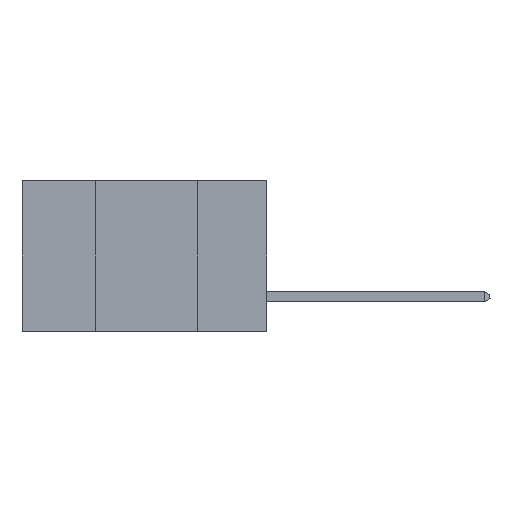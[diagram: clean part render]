
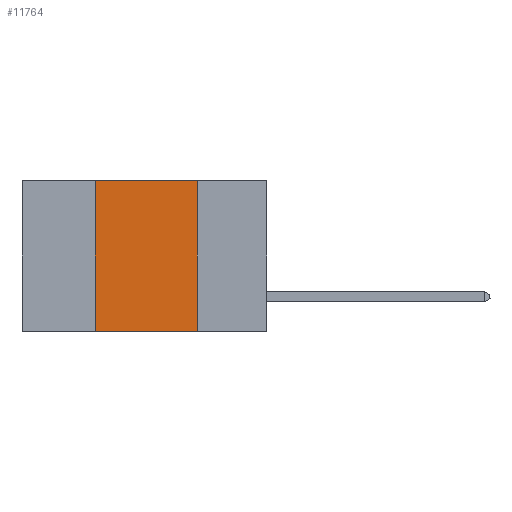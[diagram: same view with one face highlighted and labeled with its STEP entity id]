
A CAD part, left-side view. The second image highlights one B-rep face of the part: STEP entity #11764.
In plain terms, the highlighted planar face has unit normal (-1, 0, 0).
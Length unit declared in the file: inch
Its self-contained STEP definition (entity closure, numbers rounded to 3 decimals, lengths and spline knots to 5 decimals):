
#420 = PLANE ( 'NONE',  #907 ) ;
#666 = VECTOR ( 'NONE', #4192, 39.37008 ) ;
#707 = EDGE_CURVE ( 'NONE', #9899, #2850, #5835, .T. ) ;
#907 = AXIS2_PLACEMENT_3D ( 'NONE', #1849, #9413, #3931 ) ;
#1086 = ORIENTED_EDGE ( 'NONE', *, *, #3084, .F. ) ;
#1494 = EDGE_CURVE ( 'NONE', #9899, #6217, #3956, .T. ) ;
#1543 = EDGE_CURVE ( 'NONE', #2850, #6375, #12144, .T. ) ;
#1849 = CARTESIAN_POINT ( 'NONE',  ( 0., 0.6, 0. ) ) ;
#1938 = VECTOR ( 'NONE', #7849, 39.37008 ) ;
#2269 = CARTESIAN_POINT ( 'NONE',  ( 0., 0.6, -0.37 ) ) ;
#2850 = VERTEX_POINT ( 'NONE', #7704 ) ;
#2855 = CARTESIAN_POINT ( 'NONE',  ( 0., 0.17, 0. ) ) ;
#3084 = EDGE_CURVE ( 'NONE', #6375, #6217, #12260, .T. ) ;
#3342 = ORIENTED_EDGE ( 'NONE', *, *, #1494, .T. ) ;
#3931 = DIRECTION ( 'NONE',  ( 0., 0., -1. ) ) ;
#3956 = LINE ( 'NONE', #2269, #666 ) ;
#4192 = DIRECTION ( 'NONE',  ( 0., -1., 0. ) ) ;
#5398 = ORIENTED_EDGE ( 'NONE', *, *, #1543, .F. ) ;
#5835 = LINE ( 'NONE', #10474, #6326 ) ;
#6217 = VERTEX_POINT ( 'NONE', #7143 ) ;
#6326 = VECTOR ( 'NONE', #7197, 39.37008 ) ;
#6375 = VERTEX_POINT ( 'NONE', #2855 ) ;
#7088 = CARTESIAN_POINT ( 'NONE',  ( 0., 0.6, 0. ) ) ;
#7143 = CARTESIAN_POINT ( 'NONE',  ( 0., 0.17, -0.37 ) ) ;
#7197 = DIRECTION ( 'NONE',  ( 0., 0., 1. ) ) ;
#7704 = CARTESIAN_POINT ( 'NONE',  ( 0., 0.42, 0. ) ) ;
#7835 = EDGE_LOOP ( 'NONE', ( #1086, #5398, #12886, #3342 ) ) ;
#7849 = DIRECTION ( 'NONE',  ( 0., 0., -1. ) ) ;
#8139 = DIRECTION ( 'NONE',  ( 0., -1., 0. ) ) ;
#9413 = DIRECTION ( 'NONE',  ( 1., 0., 0. ) ) ;
#9899 = VERTEX_POINT ( 'NONE', #9953 ) ;
#9953 = CARTESIAN_POINT ( 'NONE',  ( 0., 0.42, -0.37 ) ) ;
#10474 = CARTESIAN_POINT ( 'NONE',  ( 0., 0.42, 0. ) ) ;
#11317 = VECTOR ( 'NONE', #8139, 39.37008 ) ;
#11764 = ADVANCED_FACE ( 'NONE', ( #13455 ), #420, .F. ) ;
#12144 = LINE ( 'NONE', #7088, #11317 ) ;
#12260 = LINE ( 'NONE', #13069, #1938 ) ;
#12886 = ORIENTED_EDGE ( 'NONE', *, *, #707, .F. ) ;
#13069 = CARTESIAN_POINT ( 'NONE',  ( 0., 0.17, 0. ) ) ;
#13455 = FACE_OUTER_BOUND ( 'NONE', #7835, .T. ) ;
